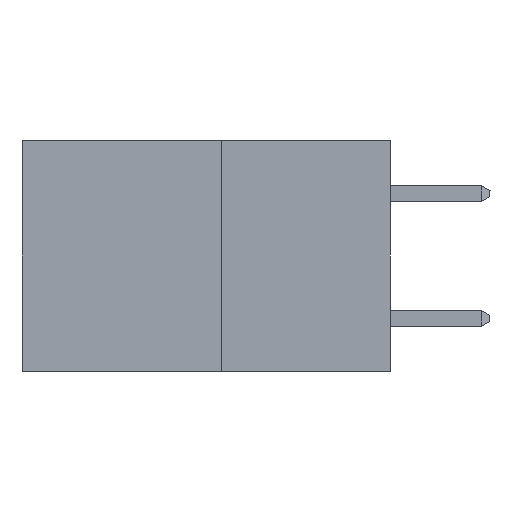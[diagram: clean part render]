
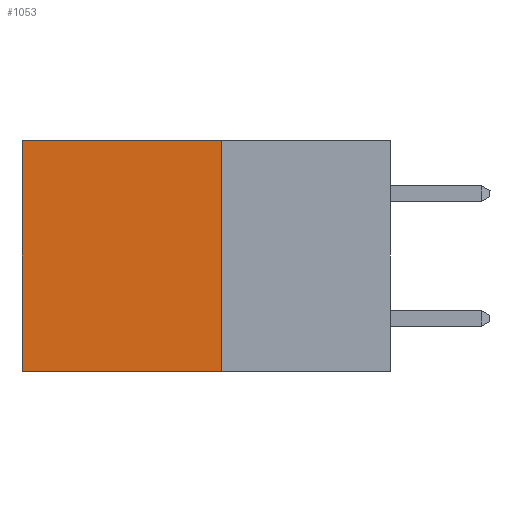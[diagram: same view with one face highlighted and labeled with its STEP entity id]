
A CAD part, left-side view. The second image highlights one B-rep face of the part: STEP entity #1053.
In plain terms, the highlighted planar face has unit normal (-1, 0, 0).
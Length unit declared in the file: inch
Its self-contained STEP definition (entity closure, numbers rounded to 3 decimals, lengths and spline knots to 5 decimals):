
#980 = EDGE_CURVE ( 'NONE', #15734, #15170, #18670, .T. ) ;
#1053 = ADVANCED_FACE ( 'NONE', ( #16801 ), #19362, .F. ) ;
#1199 = DIRECTION ( 'NONE',  ( 1., 0., 0. ) ) ;
#1265 = CARTESIAN_POINT ( 'NONE',  ( 0.277, 0.27, -0.37 ) ) ;
#2731 = VECTOR ( 'NONE', #16769, 39.37008 ) ;
#2947 = DIRECTION ( 'NONE',  ( 0., 0., -1. ) ) ;
#3294 = VECTOR ( 'NONE', #2947, 39.37008 ) ;
#3872 = VECTOR ( 'NONE', #16936, 39.37008 ) ;
#5111 = CARTESIAN_POINT ( 'NONE',  ( 0.277, 0.27, -0.37 ) ) ;
#6830 = LINE ( 'NONE', #15252, #2731 ) ;
#7028 = ORIENTED_EDGE ( 'NONE', *, *, #7373, .T. ) ;
#7373 = EDGE_CURVE ( 'NONE', #16036, #11233, #6830, .T. ) ;
#7632 = CARTESIAN_POINT ( 'NONE',  ( 0.277, 0.59, -0.37 ) ) ;
#8520 = EDGE_LOOP ( 'NONE', ( #16029, #13388, #13883, #7028 ) ) ;
#10058 = EDGE_CURVE ( 'NONE', #16036, #15734, #12017, .T. ) ;
#10531 = VECTOR ( 'NONE', #18624, 39.37008 ) ;
#11221 = CARTESIAN_POINT ( 'NONE',  ( 0.277, 0.27, -0.37 ) ) ;
#11233 = VERTEX_POINT ( 'NONE', #15612 ) ;
#12017 = LINE ( 'NONE', #13828, #3294 ) ;
#13068 = CARTESIAN_POINT ( 'NONE',  ( 0.277, 0.59, -0.37 ) ) ;
#13388 = ORIENTED_EDGE ( 'NONE', *, *, #980, .F. ) ;
#13828 = CARTESIAN_POINT ( 'NONE',  ( 0.277, 0.27, -0.37 ) ) ;
#13883 = ORIENTED_EDGE ( 'NONE', *, *, #10058, .F. ) ;
#14331 = AXIS2_PLACEMENT_3D ( 'NONE', #1265, #1199, #14667 ) ;
#14667 = DIRECTION ( 'NONE',  ( 0., 0., -1. ) ) ;
#15170 = VERTEX_POINT ( 'NONE', #13068 ) ;
#15252 = CARTESIAN_POINT ( 'NONE',  ( 0.277, 0.27, 0. ) ) ;
#15612 = CARTESIAN_POINT ( 'NONE',  ( 0.277, 0.59, 0. ) ) ;
#15734 = VERTEX_POINT ( 'NONE', #11221 ) ;
#16029 = ORIENTED_EDGE ( 'NONE', *, *, #17812, .T. ) ;
#16036 = VERTEX_POINT ( 'NONE', #18095 ) ;
#16220 = LINE ( 'NONE', #7632, #3872 ) ;
#16769 = DIRECTION ( 'NONE',  ( 0., 1., 0. ) ) ;
#16801 = FACE_OUTER_BOUND ( 'NONE', #8520, .T. ) ;
#16936 = DIRECTION ( 'NONE',  ( 0., 0., -1. ) ) ;
#17812 = EDGE_CURVE ( 'NONE', #11233, #15170, #16220, .T. ) ;
#18095 = CARTESIAN_POINT ( 'NONE',  ( 0.277, 0.27, 0. ) ) ;
#18624 = DIRECTION ( 'NONE',  ( 0., 1., 0. ) ) ;
#18670 = LINE ( 'NONE', #5111, #10531 ) ;
#19362 = PLANE ( 'NONE',  #14331 ) ;
